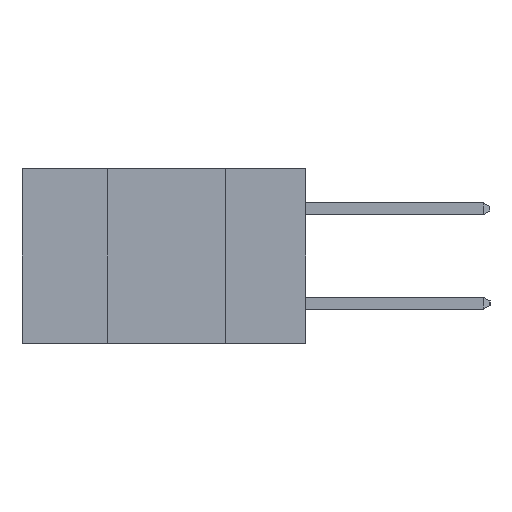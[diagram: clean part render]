
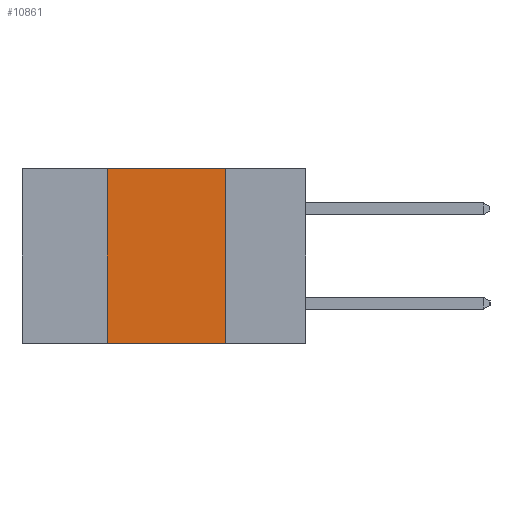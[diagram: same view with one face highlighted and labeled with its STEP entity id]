
A CAD part, left-side view. The second image highlights one B-rep face of the part: STEP entity #10861.
In plain terms, the highlighted planar face has unit normal (-1, 0, 0).
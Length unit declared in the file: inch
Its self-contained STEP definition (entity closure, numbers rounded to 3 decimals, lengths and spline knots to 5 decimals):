
#49 = LINE ( 'NONE', #2798, #5761 ) ;
#1078 = EDGE_LOOP ( 'NONE', ( #2341, #2623, #12275, #1316 ) ) ;
#1316 = ORIENTED_EDGE ( 'NONE', *, *, #8569, .T. ) ;
#1922 = VERTEX_POINT ( 'NONE', #13601 ) ;
#2177 = LINE ( 'NONE', #12206, #4904 ) ;
#2279 = LINE ( 'NONE', #7677, #7985 ) ;
#2341 = ORIENTED_EDGE ( 'NONE', *, *, #2451, .F. ) ;
#2451 = EDGE_CURVE ( 'NONE', #5577, #3493, #2279, .T. ) ;
#2623 = ORIENTED_EDGE ( 'NONE', *, *, #6887, .F. ) ;
#2652 = DIRECTION ( 'NONE',  ( 0., 0., 1. ) ) ;
#2798 = CARTESIAN_POINT ( 'NONE',  ( 0., 0.42, -0.37 ) ) ;
#3316 = CARTESIAN_POINT ( 'NONE',  ( 0., 0.17, -0.37 ) ) ;
#3321 = DIRECTION ( 'NONE',  ( 0., 0., -1. ) ) ;
#3377 = DIRECTION ( 'NONE',  ( 1., 0., 0. ) ) ;
#3493 = VERTEX_POINT ( 'NONE', #3316 ) ;
#3569 = CARTESIAN_POINT ( 'NONE',  ( 0., 0.6, 0. ) ) ;
#3799 = PLANE ( 'NONE',  #7801 ) ;
#4290 = LINE ( 'NONE', #10480, #9954 ) ;
#4904 = VECTOR ( 'NONE', #12168, 39.37008 ) ;
#5577 = VERTEX_POINT ( 'NONE', #13940 ) ;
#5730 = VERTEX_POINT ( 'NONE', #12595 ) ;
#5761 = VECTOR ( 'NONE', #2652, 39.37008 ) ;
#6887 = EDGE_CURVE ( 'NONE', #1922, #5577, #2177, .T. ) ;
#6905 = DIRECTION ( 'NONE',  ( 0., 0., -1. ) ) ;
#7677 = CARTESIAN_POINT ( 'NONE',  ( 0., 0.17, -0.37 ) ) ;
#7801 = AXIS2_PLACEMENT_3D ( 'NONE', #3569, #3377, #3321 ) ;
#7985 = VECTOR ( 'NONE', #6905, 39.37008 ) ;
#7988 = EDGE_CURVE ( 'NONE', #5730, #1922, #49, .T. ) ;
#8569 = EDGE_CURVE ( 'NONE', #5730, #3493, #4290, .T. ) ;
#9954 = VECTOR ( 'NONE', #10391, 39.37008 ) ;
#10391 = DIRECTION ( 'NONE',  ( 0., -1., 0. ) ) ;
#10480 = CARTESIAN_POINT ( 'NONE',  ( 0., 0.6, -0.37 ) ) ;
#10861 = ADVANCED_FACE ( 'NONE', ( #11660 ), #3799, .F. ) ;
#11660 = FACE_OUTER_BOUND ( 'NONE', #1078, .T. ) ;
#12168 = DIRECTION ( 'NONE',  ( 0., -1., 0. ) ) ;
#12206 = CARTESIAN_POINT ( 'NONE',  ( 0., 0.6, 0. ) ) ;
#12275 = ORIENTED_EDGE ( 'NONE', *, *, #7988, .F. ) ;
#12595 = CARTESIAN_POINT ( 'NONE',  ( 0., 0.42, -0.37 ) ) ;
#13601 = CARTESIAN_POINT ( 'NONE',  ( 0., 0.42, 0. ) ) ;
#13940 = CARTESIAN_POINT ( 'NONE',  ( 0., 0.17, 0. ) ) ;
